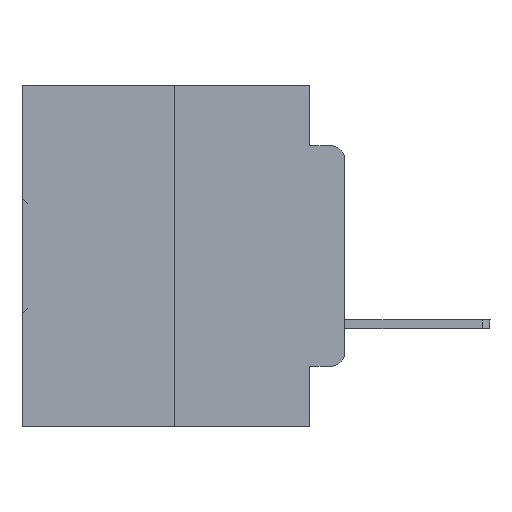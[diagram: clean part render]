
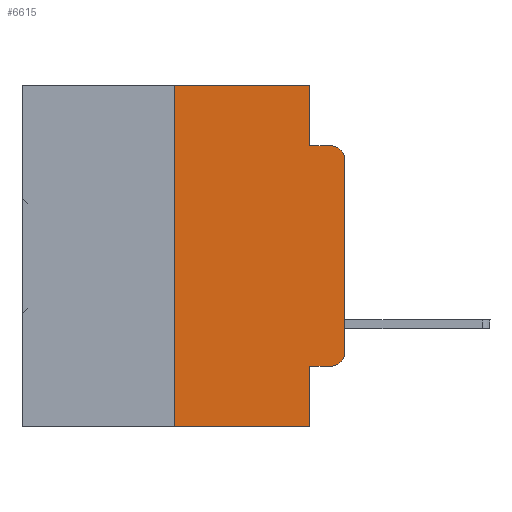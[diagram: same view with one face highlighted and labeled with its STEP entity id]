
A CAD part, left-side view. The second image highlights one B-rep face of the part: STEP entity #6615.
In plain terms, the highlighted planar face has unit normal (-1, 0, 0).
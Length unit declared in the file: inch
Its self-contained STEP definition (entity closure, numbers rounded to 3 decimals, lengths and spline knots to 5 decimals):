
#1136 = DIRECTION ( 'NONE',  ( 0., -1., 0. ) ) ;
#1306 = AXIS2_PLACEMENT_3D ( 'NONE', #18331, #18154, #7392 ) ;
#1745 = AXIS2_PLACEMENT_3D ( 'NONE', #24523, #7926, #24177 ) ;
#1807 = VERTEX_POINT ( 'NONE', #9163 ) ;
#2100 = ORIENTED_EDGE ( 'NONE', *, *, #24857, .F. ) ;
#2435 = VERTEX_POINT ( 'NONE', #34760 ) ;
#2742 = CIRCLE ( 'NONE', #15703, 0.02 ) ;
#2805 = VECTOR ( 'NONE', #20511, 39.37008 ) ;
#3099 = ORIENTED_EDGE ( 'NONE', *, *, #23143, .F. ) ;
#3780 = LINE ( 'NONE', #33486, #27010 ) ;
#3927 = VERTEX_POINT ( 'NONE', #17404 ) ;
#4028 = VECTOR ( 'NONE', #20324, 39.37008 ) ;
#4059 = CARTESIAN_POINT ( 'NONE',  ( 0., 0.051, 0. ) ) ;
#4936 = DIRECTION ( 'NONE',  ( 0., -1., 0. ) ) ;
#5096 = VECTOR ( 'NONE', #17323, 39.37008 ) ;
#5185 = VERTEX_POINT ( 'NONE', #27919 ) ;
#6224 = VECTOR ( 'NONE', #12451, 39.37008 ) ;
#6615 = ADVANCED_FACE ( 'NONE', ( #34635 ), #31619, .F. ) ;
#6891 = LINE ( 'NONE', #14673, #2805 ) ;
#7153 = DIRECTION ( 'NONE',  ( 0., 0., 1. ) ) ;
#7392 = DIRECTION ( 'NONE',  ( 0., 0., -1. ) ) ;
#7926 = DIRECTION ( 'NONE',  ( -1., 0., 0. ) ) ;
#9163 = CARTESIAN_POINT ( 'NONE',  ( 0., 0.02, -0.0885 ) ) ;
#9481 = ORIENTED_EDGE ( 'NONE', *, *, #13294, .T. ) ;
#9873 = VERTEX_POINT ( 'NONE', #32561 ) ;
#10291 = ORIENTED_EDGE ( 'NONE', *, *, #15092, .T. ) ;
#11075 = LINE ( 'NONE', #24850, #31516 ) ;
#11321 = EDGE_LOOP ( 'NONE', ( #21198, #27931, #28149, #33086, #3099, #23049, #9481, #2100, #10291, #34930 ) ) ;
#12341 = VERTEX_POINT ( 'NONE', #25125 ) ;
#12451 = DIRECTION ( 'NONE',  ( 0., -1., 0. ) ) ;
#12648 = LINE ( 'NONE', #25890, #15352 ) ;
#13145 = EDGE_CURVE ( 'NONE', #15892, #1807, #2742, .T. ) ;
#13294 = EDGE_CURVE ( 'NONE', #25531, #9873, #3780, .T. ) ;
#13574 = CARTESIAN_POINT ( 'NONE',  ( 0., 0.02, -0.1085 ) ) ;
#14673 = CARTESIAN_POINT ( 'NONE',  ( 0., 0.473, 0. ) ) ;
#15092 = EDGE_CURVE ( 'NONE', #12341, #2435, #29715, .T. ) ;
#15352 = VECTOR ( 'NONE', #7153, 39.37008 ) ;
#15703 = AXIS2_PLACEMENT_3D ( 'NONE', #13574, #17039, #27845 ) ;
#15892 = VERTEX_POINT ( 'NONE', #28415 ) ;
#16315 = EDGE_CURVE ( 'NONE', #2435, #27163, #23112, .T. ) ;
#17039 = DIRECTION ( 'NONE',  ( -1., 0., 0. ) ) ;
#17323 = DIRECTION ( 'NONE',  ( 0., 0., -1. ) ) ;
#17404 = CARTESIAN_POINT ( 'NONE',  ( 0., 0.25, 0. ) ) ;
#18023 = LINE ( 'NONE', #28485, #5096 ) ;
#18154 = DIRECTION ( 'NONE',  ( 1., 0., 0. ) ) ;
#18331 = CARTESIAN_POINT ( 'NONE',  ( 0., 0.473, 0. ) ) ;
#20136 = LINE ( 'NONE', #4059, #4028 ) ;
#20324 = DIRECTION ( 'NONE',  ( 0., 0., -1. ) ) ;
#20511 = DIRECTION ( 'NONE',  ( 0., -1., 0. ) ) ;
#21198 = ORIENTED_EDGE ( 'NONE', *, *, #29983, .T. ) ;
#21717 = CARTESIAN_POINT ( 'NONE',  ( 0., 0.051, -0.0885 ) ) ;
#22158 = CARTESIAN_POINT ( 'NONE',  ( 0., 0., -0.3915 ) ) ;
#23049 = ORIENTED_EDGE ( 'NONE', *, *, #26930, .F. ) ;
#23112 = CIRCLE ( 'NONE', #1745, 0.02 ) ;
#23143 = EDGE_CURVE ( 'NONE', #3927, #5185, #6891, .T. ) ;
#24118 = CARTESIAN_POINT ( 'NONE',  ( 0., 0.051, -0.0885 ) ) ;
#24177 = DIRECTION ( 'NONE',  ( 0., 0., -1. ) ) ;
#24499 = DIRECTION ( 'NONE',  ( 0., 0., 1. ) ) ;
#24523 = CARTESIAN_POINT ( 'NONE',  ( 0., 0.02, -0.3915 ) ) ;
#24850 = CARTESIAN_POINT ( 'NONE',  ( 0., 0., 0. ) ) ;
#24857 = EDGE_CURVE ( 'NONE', #12341, #9873, #20136, .T. ) ;
#24950 = EDGE_CURVE ( 'NONE', #31382, #1807, #29681, .T. ) ;
#25125 = CARTESIAN_POINT ( 'NONE',  ( 0., 0.051, -0.4115 ) ) ;
#25531 = VERTEX_POINT ( 'NONE', #29997 ) ;
#25875 = CARTESIAN_POINT ( 'NONE',  ( 0., 0.051, -0.4115 ) ) ;
#25890 = CARTESIAN_POINT ( 'NONE',  ( 0., 0.25, 0. ) ) ;
#26032 = VECTOR ( 'NONE', #4936, 39.37008 ) ;
#26930 = EDGE_CURVE ( 'NONE', #25531, #3927, #12648, .T. ) ;
#27010 = VECTOR ( 'NONE', #1136, 39.37008 ) ;
#27163 = VERTEX_POINT ( 'NONE', #22158 ) ;
#27845 = DIRECTION ( 'NONE',  ( 0., 0., -1. ) ) ;
#27919 = CARTESIAN_POINT ( 'NONE',  ( 0., 0.051, 0. ) ) ;
#27931 = ORIENTED_EDGE ( 'NONE', *, *, #13145, .T. ) ;
#28149 = ORIENTED_EDGE ( 'NONE', *, *, #24950, .F. ) ;
#28415 = CARTESIAN_POINT ( 'NONE',  ( 0., 0., -0.1085 ) ) ;
#28485 = CARTESIAN_POINT ( 'NONE',  ( 0., 0.051, 0. ) ) ;
#29681 = LINE ( 'NONE', #21717, #26032 ) ;
#29715 = LINE ( 'NONE', #25875, #6224 ) ;
#29983 = EDGE_CURVE ( 'NONE', #27163, #15892, #11075, .T. ) ;
#29997 = CARTESIAN_POINT ( 'NONE',  ( 0., 0.25, -0.5 ) ) ;
#31382 = VERTEX_POINT ( 'NONE', #24118 ) ;
#31516 = VECTOR ( 'NONE', #24499, 39.37008 ) ;
#31619 = PLANE ( 'NONE',  #1306 ) ;
#32561 = CARTESIAN_POINT ( 'NONE',  ( 0., 0.051, -0.5 ) ) ;
#33086 = ORIENTED_EDGE ( 'NONE', *, *, #33934, .F. ) ;
#33486 = CARTESIAN_POINT ( 'NONE',  ( 0., 0.473, -0.5 ) ) ;
#33934 = EDGE_CURVE ( 'NONE', #5185, #31382, #18023, .T. ) ;
#34635 = FACE_OUTER_BOUND ( 'NONE', #11321, .T. ) ;
#34760 = CARTESIAN_POINT ( 'NONE',  ( 0., 0.02, -0.4115 ) ) ;
#34930 = ORIENTED_EDGE ( 'NONE', *, *, #16315, .T. ) ;
